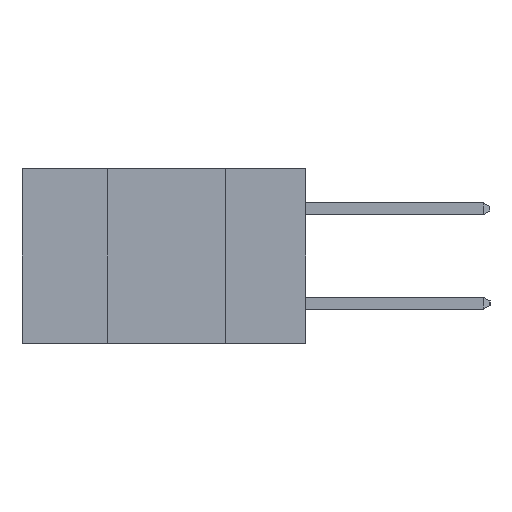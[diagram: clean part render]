
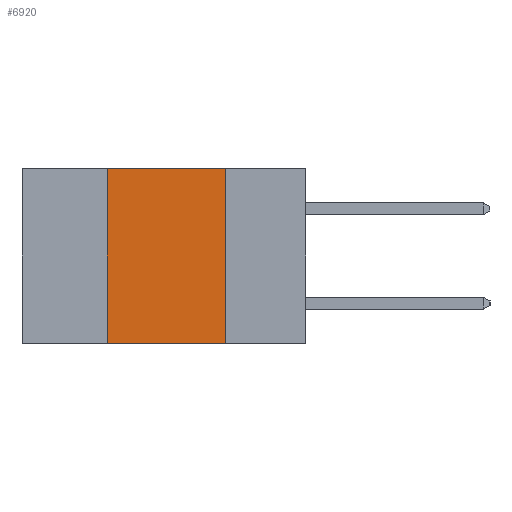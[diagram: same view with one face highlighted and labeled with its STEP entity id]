
A CAD part, left-side view. The second image highlights one B-rep face of the part: STEP entity #6920.
In plain terms, the highlighted planar face has unit normal (-1, 0, 0).
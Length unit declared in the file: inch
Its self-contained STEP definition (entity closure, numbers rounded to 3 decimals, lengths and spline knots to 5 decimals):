
#1256 = CARTESIAN_POINT ( 'NONE',  ( 0., 0.17, -0.37 ) ) ;
#1353 = VERTEX_POINT ( 'NONE', #5539 ) ;
#1500 = DIRECTION ( 'NONE',  ( 0., 0., -1. ) ) ;
#1861 = VERTEX_POINT ( 'NONE', #5085 ) ;
#2159 = VECTOR ( 'NONE', #6728, 39.37008 ) ;
#3550 = CARTESIAN_POINT ( 'NONE',  ( 0., 0.6, -0.37 ) ) ;
#3837 = EDGE_CURVE ( 'NONE', #1353, #9913, #6857, .T. ) ;
#4282 = CARTESIAN_POINT ( 'NONE',  ( 0., 0.6, 0. ) ) ;
#4607 = DIRECTION ( 'NONE',  ( 0., 0., 1. ) ) ;
#4739 = LINE ( 'NONE', #4282, #2159 ) ;
#4955 = VECTOR ( 'NONE', #4607, 39.37008 ) ;
#4987 = CARTESIAN_POINT ( 'NONE',  ( 0., 0.17, 0. ) ) ;
#5033 = AXIS2_PLACEMENT_3D ( 'NONE', #10557, #6553, #1500 ) ;
#5085 = CARTESIAN_POINT ( 'NONE',  ( 0., 0.17, -0.37 ) ) ;
#5532 = EDGE_LOOP ( 'NONE', ( #7511, #5894, #6157, #6504 ) ) ;
#5539 = CARTESIAN_POINT ( 'NONE',  ( 0., 0.42, -0.37 ) ) ;
#5720 = EDGE_CURVE ( 'NONE', #1353, #1861, #9206, .T. ) ;
#5743 = PLANE ( 'NONE',  #5033 ) ;
#5894 = ORIENTED_EDGE ( 'NONE', *, *, #8202, .F. ) ;
#6157 = ORIENTED_EDGE ( 'NONE', *, *, #3837, .F. ) ;
#6164 = CARTESIAN_POINT ( 'NONE',  ( 0., 0.42, 0. ) ) ;
#6256 = VERTEX_POINT ( 'NONE', #4987 ) ;
#6504 = ORIENTED_EDGE ( 'NONE', *, *, #5720, .T. ) ;
#6553 = DIRECTION ( 'NONE',  ( 1., 0., 0. ) ) ;
#6728 = DIRECTION ( 'NONE',  ( 0., -1., 0. ) ) ;
#6857 = LINE ( 'NONE', #7805, #4955 ) ;
#6920 = ADVANCED_FACE ( 'NONE', ( #9556 ), #5743, .F. ) ;
#7060 = VECTOR ( 'NONE', #7683, 39.37008 ) ;
#7114 = DIRECTION ( 'NONE',  ( 0., 0., -1. ) ) ;
#7511 = ORIENTED_EDGE ( 'NONE', *, *, #8551, .F. ) ;
#7683 = DIRECTION ( 'NONE',  ( 0., -1., 0. ) ) ;
#7805 = CARTESIAN_POINT ( 'NONE',  ( 0., 0.42, -0.37 ) ) ;
#8202 = EDGE_CURVE ( 'NONE', #9913, #6256, #4739, .T. ) ;
#8551 = EDGE_CURVE ( 'NONE', #6256, #1861, #9800, .T. ) ;
#9206 = LINE ( 'NONE', #3550, #7060 ) ;
#9556 = FACE_OUTER_BOUND ( 'NONE', #5532, .T. ) ;
#9800 = LINE ( 'NONE', #1256, #10040 ) ;
#9913 = VERTEX_POINT ( 'NONE', #6164 ) ;
#10040 = VECTOR ( 'NONE', #7114, 39.37008 ) ;
#10557 = CARTESIAN_POINT ( 'NONE',  ( 0., 0.6, 0. ) ) ;
